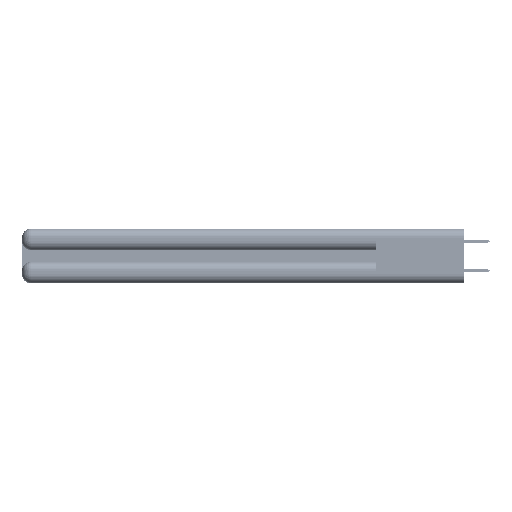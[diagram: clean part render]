
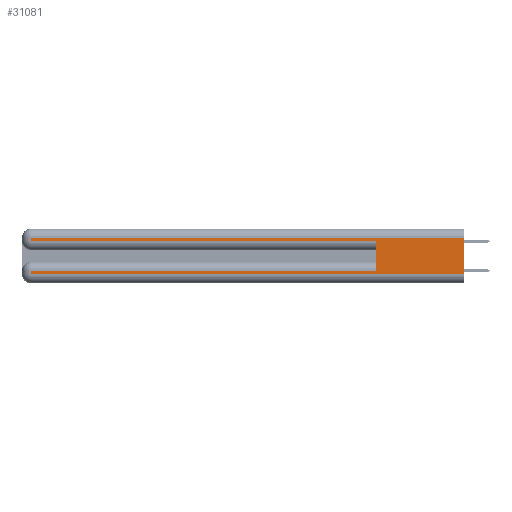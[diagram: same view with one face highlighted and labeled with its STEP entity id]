
A CAD part, left-side view. The second image highlights one B-rep face of the part: STEP entity #31081.
In plain terms, the highlighted planar face has unit normal (-1, 0, 0).
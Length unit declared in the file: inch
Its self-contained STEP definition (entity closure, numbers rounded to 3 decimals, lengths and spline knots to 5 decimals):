
#48 = ORIENTED_EDGE ( 'NONE', *, *, #5620, .T. ) ;
#303 = CARTESIAN_POINT ( 'NONE',  ( 0., 0.6, 0.145 ) ) ;
#519 = DIRECTION ( 'NONE',  ( 1., 0., 0. ) ) ;
#675 = VECTOR ( 'NONE', #16144, 39.37008 ) ;
#887 = EDGE_CURVE ( 'NONE', #7448, #39956, #36398, .T. ) ;
#1224 = CARTESIAN_POINT ( 'NONE',  ( 0., 2.94, 0.285 ) ) ;
#3167 = CARTESIAN_POINT ( 'NONE',  ( 0., 2.94, 0.37 ) ) ;
#3256 = ORIENTED_EDGE ( 'NONE', *, *, #5930, .T. ) ;
#3427 = DIRECTION ( 'NONE',  ( 0., -1., 0. ) ) ;
#3995 = LINE ( 'NONE', #32596, #45451 ) ;
#4417 = DIRECTION ( 'NONE',  ( 0., 0., -1. ) ) ;
#5620 = EDGE_CURVE ( 'NONE', #23498, #40974, #43221, .T. ) ;
#5930 = EDGE_CURVE ( 'NONE', #29073, #12764, #17499, .T. ) ;
#6723 = CARTESIAN_POINT ( 'NONE',  ( 0., 0., 0.06 ) ) ;
#7448 = VERTEX_POINT ( 'NONE', #1224 ) ;
#8321 = VERTEX_POINT ( 'NONE', #26530 ) ;
#9294 = DIRECTION ( 'NONE',  ( 0., 1., 0. ) ) ;
#12082 = CARTESIAN_POINT ( 'NONE',  ( 0., 0., 0.31 ) ) ;
#12535 = PLANE ( 'NONE',  #14176 ) ;
#12760 = LINE ( 'NONE', #3167, #22224 ) ;
#12764 = VERTEX_POINT ( 'NONE', #6723 ) ;
#14176 = AXIS2_PLACEMENT_3D ( 'NONE', #24656, #519, #28745 ) ;
#15052 = VECTOR ( 'NONE', #27250, 39.37008 ) ;
#15144 = FACE_OUTER_BOUND ( 'NONE', #47600, .T. ) ;
#15210 = LINE ( 'NONE', #36972, #35315 ) ;
#16144 = DIRECTION ( 'NONE',  ( 0., 1., 0. ) ) ;
#16230 = VECTOR ( 'NONE', #3427, 39.37008 ) ;
#16558 = DIRECTION ( 'NONE',  ( 0., 0., 1. ) ) ;
#17093 = ORIENTED_EDGE ( 'NONE', *, *, #27261, .F. ) ;
#17499 = LINE ( 'NONE', #31625, #16230 ) ;
#20830 = ORIENTED_EDGE ( 'NONE', *, *, #36668, .T. ) ;
#22153 = EDGE_CURVE ( 'NONE', #40974, #29073, #12760, .T. ) ;
#22224 = VECTOR ( 'NONE', #43381, 39.37008 ) ;
#22737 = ORIENTED_EDGE ( 'NONE', *, *, #887, .T. ) ;
#23165 = CARTESIAN_POINT ( 'NONE',  ( 0., 0., 0.285 ) ) ;
#23498 = VERTEX_POINT ( 'NONE', #49828 ) ;
#24132 = CARTESIAN_POINT ( 'NONE',  ( 0., 2.94, 0.06 ) ) ;
#24656 = CARTESIAN_POINT ( 'NONE',  ( 0., 0., 0.37 ) ) ;
#25034 = DIRECTION ( 'NONE',  ( 0., 0., -1. ) ) ;
#26485 = ORIENTED_EDGE ( 'NONE', *, *, #48407, .F. ) ;
#26530 = CARTESIAN_POINT ( 'NONE',  ( 0., 0., 0.31 ) ) ;
#26916 = LINE ( 'NONE', #303, #45628 ) ;
#27250 = DIRECTION ( 'NONE',  ( 0., -1., 0. ) ) ;
#27261 = EDGE_CURVE ( 'NONE', #23498, #39956, #26916, .T. ) ;
#28745 = DIRECTION ( 'NONE',  ( 0., 0., -1. ) ) ;
#29073 = VERTEX_POINT ( 'NONE', #24132 ) ;
#31081 = ADVANCED_FACE ( 'NONE', ( #15144 ), #12535, .F. ) ;
#31365 = VECTOR ( 'NONE', #9294, 39.37008 ) ;
#31610 = VERTEX_POINT ( 'NONE', #38370 ) ;
#31625 = CARTESIAN_POINT ( 'NONE',  ( 0., 0., 0.06 ) ) ;
#32596 = CARTESIAN_POINT ( 'NONE',  ( 0., 0., 0.37 ) ) ;
#32818 = LINE ( 'NONE', #12082, #675 ) ;
#33051 = CARTESIAN_POINT ( 'NONE',  ( 0., 0.6, 0.285 ) ) ;
#35315 = VECTOR ( 'NONE', #25034, 39.37008 ) ;
#36398 = LINE ( 'NONE', #23165, #15052 ) ;
#36668 = EDGE_CURVE ( 'NONE', #31610, #7448, #15210, .T. ) ;
#36972 = CARTESIAN_POINT ( 'NONE',  ( 0., 2.94, 0.37 ) ) ;
#37425 = CARTESIAN_POINT ( 'NONE',  ( 0., 0., 0.085 ) ) ;
#38370 = CARTESIAN_POINT ( 'NONE',  ( 0., 2.94, 0.31 ) ) ;
#39956 = VERTEX_POINT ( 'NONE', #33051 ) ;
#40781 = CARTESIAN_POINT ( 'NONE',  ( 0., 2.94, 0.085 ) ) ;
#40883 = ORIENTED_EDGE ( 'NONE', *, *, #46041, .T. ) ;
#40974 = VERTEX_POINT ( 'NONE', #40781 ) ;
#42238 = ORIENTED_EDGE ( 'NONE', *, *, #22153, .T. ) ;
#43221 = LINE ( 'NONE', #37425, #31365 ) ;
#43381 = DIRECTION ( 'NONE',  ( 0., 0., -1. ) ) ;
#45451 = VECTOR ( 'NONE', #4417, 39.37008 ) ;
#45628 = VECTOR ( 'NONE', #16558, 39.37008 ) ;
#46041 = EDGE_CURVE ( 'NONE', #8321, #31610, #32818, .T. ) ;
#47600 = EDGE_LOOP ( 'NONE', ( #26485, #40883, #20830, #22737, #17093, #48, #42238, #3256 ) ) ;
#48407 = EDGE_CURVE ( 'NONE', #8321, #12764, #3995, .T. ) ;
#49828 = CARTESIAN_POINT ( 'NONE',  ( 0., 0.6, 0.085 ) ) ;
